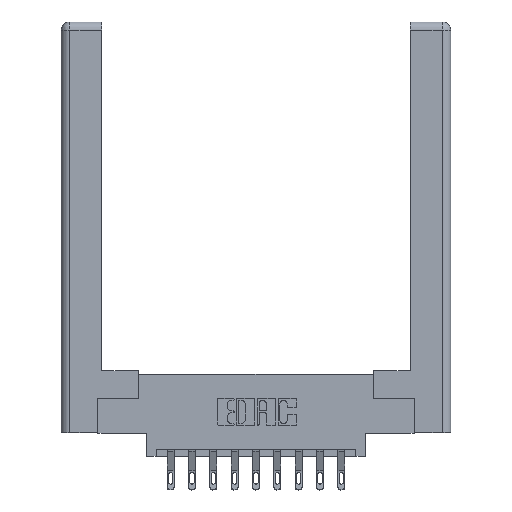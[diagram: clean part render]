
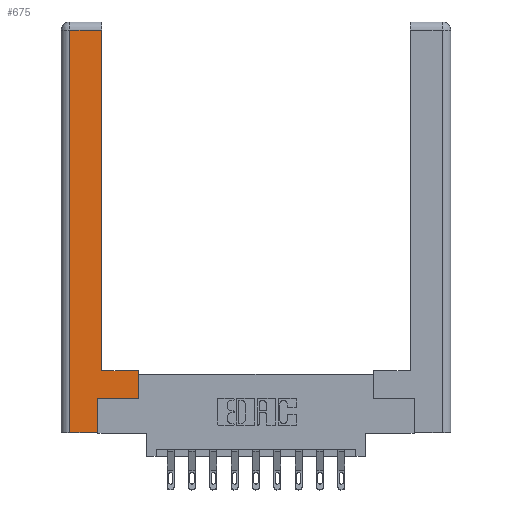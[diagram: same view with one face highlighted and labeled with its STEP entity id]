
A CAD part, top view. The second image highlights one B-rep face of the part: STEP entity #675.
In plain terms, the highlighted planar face has unit normal (0, 0, 1).
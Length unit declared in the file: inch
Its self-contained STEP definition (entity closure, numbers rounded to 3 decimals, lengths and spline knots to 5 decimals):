
#148 = CARTESIAN_POINT ( 'NONE',  ( 0.565, 0.245, 0. ) ) ;
#576 = CARTESIAN_POINT ( 'NONE',  ( 0.265, 0., 0. ) ) ;
#675 = ADVANCED_FACE ( 'NONE', ( #878 ), #11489, .F. ) ;
#732 = CARTESIAN_POINT ( 'NONE',  ( 0.0615, 2.94, 0. ) ) ;
#878 = FACE_OUTER_BOUND ( 'NONE', #10270, .T. ) ;
#1506 = DIRECTION ( 'NONE',  ( 0., 0., -1. ) ) ;
#1519 = AXIS2_PLACEMENT_3D ( 'NONE', #3591, #1506, #9296 ) ;
#1520 = CARTESIAN_POINT ( 'NONE',  ( 0.565, 0.45, 0. ) ) ;
#1602 = EDGE_CURVE ( 'NONE', #9561, #2109, #14265, .T. ) ;
#1695 = ORIENTED_EDGE ( 'NONE', *, *, #9943, .T. ) ;
#1743 = DIRECTION ( 'NONE',  ( -1., 0., 0. ) ) ;
#2109 = VERTEX_POINT ( 'NONE', #7167 ) ;
#2125 = DIRECTION ( 'NONE',  ( -1., 0., 0. ) ) ;
#2308 = CARTESIAN_POINT ( 'NONE',  ( 0.265, 0., 0. ) ) ;
#3504 = CARTESIAN_POINT ( 'NONE',  ( 0.565, 0.245, 0. ) ) ;
#3591 = CARTESIAN_POINT ( 'NONE',  ( 0., 0., 0. ) ) ;
#3850 = ORIENTED_EDGE ( 'NONE', *, *, #7812, .T. ) ;
#4437 = LINE ( 'NONE', #12764, #10549 ) ;
#4597 = EDGE_CURVE ( 'NONE', #8788, #7850, #10904, .T. ) ;
#4869 = VERTEX_POINT ( 'NONE', #5060 ) ;
#4930 = EDGE_CURVE ( 'NONE', #13255, #9112, #4437, .T. ) ;
#4999 = DIRECTION ( 'NONE',  ( 1., 0., 0. ) ) ;
#5003 = CARTESIAN_POINT ( 'NONE',  ( 0.295, 0.45, 0. ) ) ;
#5060 = CARTESIAN_POINT ( 'NONE',  ( 0.295, 2.94, 0. ) ) ;
#5180 = LINE ( 'NONE', #732, #12999 ) ;
#5193 = CARTESIAN_POINT ( 'NONE',  ( 0.565, 0.45, 0. ) ) ;
#5533 = ORIENTED_EDGE ( 'NONE', *, *, #12759, .T. ) ;
#6110 = ORIENTED_EDGE ( 'NONE', *, *, #12721, .T. ) ;
#6280 = CARTESIAN_POINT ( 'NONE',  ( 0.265, 0.245, 0. ) ) ;
#7167 = CARTESIAN_POINT ( 'NONE',  ( 0.265, 0.245, 0. ) ) ;
#7174 = DIRECTION ( 'NONE',  ( 0., 1., 0. ) ) ;
#7195 = DIRECTION ( 'NONE',  ( 0., 1., 0. ) ) ;
#7349 = LINE ( 'NONE', #9427, #12727 ) ;
#7812 = EDGE_CURVE ( 'NONE', #7850, #4869, #7349, .T. ) ;
#7850 = VERTEX_POINT ( 'NONE', #5003 ) ;
#7929 = VECTOR ( 'NONE', #1743, 39.37008 ) ;
#8157 = CARTESIAN_POINT ( 'NONE',  ( 0.0615, 2.94, 0. ) ) ;
#8788 = VERTEX_POINT ( 'NONE', #5193 ) ;
#8889 = ORIENTED_EDGE ( 'NONE', *, *, #4930, .T. ) ;
#9072 = ORIENTED_EDGE ( 'NONE', *, *, #1602, .T. ) ;
#9112 = VERTEX_POINT ( 'NONE', #11943 ) ;
#9296 = DIRECTION ( 'NONE',  ( -1., 0., 0. ) ) ;
#9427 = CARTESIAN_POINT ( 'NONE',  ( 0.295, 3., 0. ) ) ;
#9561 = VERTEX_POINT ( 'NONE', #2308 ) ;
#9680 = ORIENTED_EDGE ( 'NONE', *, *, #10980, .T. ) ;
#9752 = ORIENTED_EDGE ( 'NONE', *, *, #4597, .T. ) ;
#9943 = EDGE_CURVE ( 'NONE', #9112, #9561, #10247, .T. ) ;
#10247 = LINE ( 'NONE', #576, #14076 ) ;
#10270 = EDGE_LOOP ( 'NONE', ( #3850, #9680, #8889, #1695, #9072, #6110, #5533, #9752 ) ) ;
#10527 = VECTOR ( 'NONE', #7174, 39.37008 ) ;
#10549 = VECTOR ( 'NONE', #13788, 39.37008 ) ;
#10555 = DIRECTION ( 'NONE',  ( 1., 0., 0. ) ) ;
#10593 = DIRECTION ( 'NONE',  ( 0., 1., 0. ) ) ;
#10699 = LINE ( 'NONE', #3504, #14171 ) ;
#10904 = LINE ( 'NONE', #13586, #7929 ) ;
#10980 = EDGE_CURVE ( 'NONE', #4869, #13255, #5180, .T. ) ;
#11483 = VECTOR ( 'NONE', #7195, 39.37008 ) ;
#11489 = PLANE ( 'NONE',  #1519 ) ;
#11943 = CARTESIAN_POINT ( 'NONE',  ( 0.0615, 0., 0. ) ) ;
#12721 = EDGE_CURVE ( 'NONE', #2109, #13816, #10699, .T. ) ;
#12727 = VECTOR ( 'NONE', #10593, 39.37008 ) ;
#12759 = EDGE_CURVE ( 'NONE', #13816, #8788, #13817, .T. ) ;
#12764 = CARTESIAN_POINT ( 'NONE',  ( 0.0615, 0., 0. ) ) ;
#12999 = VECTOR ( 'NONE', #2125, 39.37008 ) ;
#13255 = VERTEX_POINT ( 'NONE', #8157 ) ;
#13586 = CARTESIAN_POINT ( 'NONE',  ( 0.295, 0.45, 0. ) ) ;
#13788 = DIRECTION ( 'NONE',  ( 0., -1., 0. ) ) ;
#13816 = VERTEX_POINT ( 'NONE', #148 ) ;
#13817 = LINE ( 'NONE', #1520, #10527 ) ;
#14076 = VECTOR ( 'NONE', #10555, 39.37008 ) ;
#14171 = VECTOR ( 'NONE', #4999, 39.37008 ) ;
#14265 = LINE ( 'NONE', #6280, #11483 ) ;
